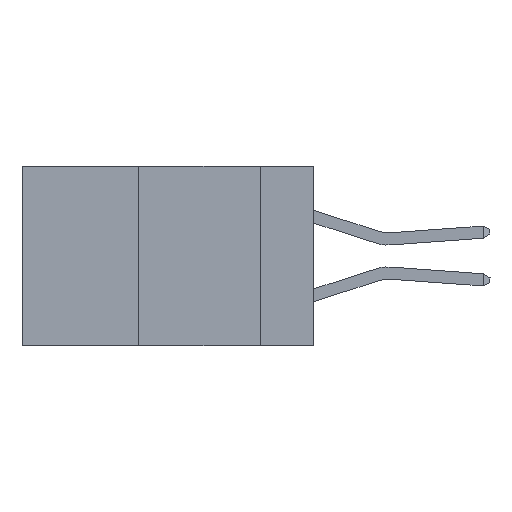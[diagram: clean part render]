
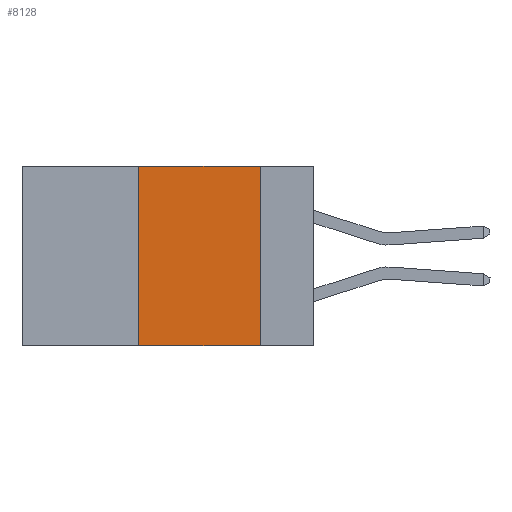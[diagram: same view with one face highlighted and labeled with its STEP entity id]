
A CAD part, left-side view. The second image highlights one B-rep face of the part: STEP entity #8128.
In plain terms, the highlighted planar face has unit normal (-1, 0, 0).
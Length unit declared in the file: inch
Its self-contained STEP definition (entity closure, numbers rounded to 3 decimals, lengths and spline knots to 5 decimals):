
#505 = ORIENTED_EDGE ( 'NONE', *, *, #1212, .F. ) ;
#715 = DIRECTION ( 'NONE',  ( 0., 0., -1. ) ) ;
#786 = CARTESIAN_POINT ( 'NONE',  ( 0., 0.11, 0. ) ) ;
#802 = CARTESIAN_POINT ( 'NONE',  ( 0., 0.11, 0. ) ) ;
#1194 = LINE ( 'NONE', #7651, #4986 ) ;
#1212 = EDGE_CURVE ( 'NONE', #2200, #5681, #1194, .T. ) ;
#1245 = VECTOR ( 'NONE', #3357, 39.37008 ) ;
#1899 = VERTEX_POINT ( 'NONE', #5765 ) ;
#2106 = CARTESIAN_POINT ( 'NONE',  ( 0., 0.36, 0. ) ) ;
#2151 = CARTESIAN_POINT ( 'NONE',  ( 0., 0.11, -0.37 ) ) ;
#2200 = VERTEX_POINT ( 'NONE', #2106 ) ;
#2416 = CARTESIAN_POINT ( 'NONE',  ( 0., 0.36, 0. ) ) ;
#2600 = VECTOR ( 'NONE', #715, 39.37008 ) ;
#3179 = VECTOR ( 'NONE', #5078, 39.37008 ) ;
#3246 = ORIENTED_EDGE ( 'NONE', *, *, #8003, .T. ) ;
#3357 = DIRECTION ( 'NONE',  ( 0., -1., 0. ) ) ;
#3360 = LINE ( 'NONE', #5834, #1245 ) ;
#3780 = DIRECTION ( 'NONE',  ( 1., 0., 0. ) ) ;
#4038 = EDGE_LOOP ( 'NONE', ( #8307, #505, #8869, #3246 ) ) ;
#4257 = EDGE_CURVE ( 'NONE', #5681, #5903, #6103, .T. ) ;
#4620 = FACE_OUTER_BOUND ( 'NONE', #4038, .T. ) ;
#4986 = VECTOR ( 'NONE', #8277, 39.37008 ) ;
#5078 = DIRECTION ( 'NONE',  ( 0., 0., 1. ) ) ;
#5681 = VERTEX_POINT ( 'NONE', #802 ) ;
#5765 = CARTESIAN_POINT ( 'NONE',  ( 0., 0.36, -0.37 ) ) ;
#5834 = CARTESIAN_POINT ( 'NONE',  ( 0., 0.6, -0.37 ) ) ;
#5888 = AXIS2_PLACEMENT_3D ( 'NONE', #7801, #3780, #8419 ) ;
#5903 = VERTEX_POINT ( 'NONE', #2151 ) ;
#6045 = EDGE_CURVE ( 'NONE', #1899, #2200, #8511, .T. ) ;
#6103 = LINE ( 'NONE', #786, #2600 ) ;
#6436 = PLANE ( 'NONE',  #5888 ) ;
#7651 = CARTESIAN_POINT ( 'NONE',  ( 0., 0.6, 0. ) ) ;
#7801 = CARTESIAN_POINT ( 'NONE',  ( 0., 0.6, 0. ) ) ;
#8003 = EDGE_CURVE ( 'NONE', #1899, #5903, #3360, .T. ) ;
#8128 = ADVANCED_FACE ( 'NONE', ( #4620 ), #6436, .F. ) ;
#8277 = DIRECTION ( 'NONE',  ( 0., -1., 0. ) ) ;
#8307 = ORIENTED_EDGE ( 'NONE', *, *, #4257, .F. ) ;
#8419 = DIRECTION ( 'NONE',  ( 0., 0., -1. ) ) ;
#8511 = LINE ( 'NONE', #2416, #3179 ) ;
#8869 = ORIENTED_EDGE ( 'NONE', *, *, #6045, .F. ) ;
